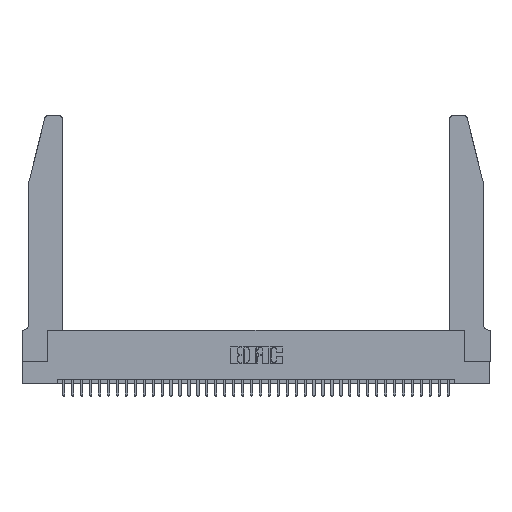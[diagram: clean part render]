
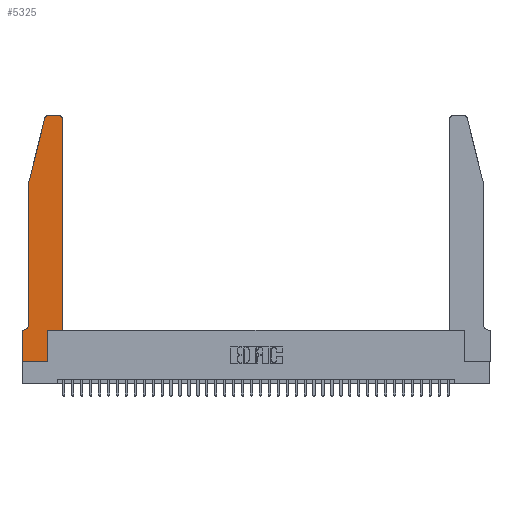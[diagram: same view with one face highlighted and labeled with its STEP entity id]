
A CAD part, top view. The second image highlights one B-rep face of the part: STEP entity #5325.
In plain terms, the highlighted planar face has unit normal (0, 0, 1).
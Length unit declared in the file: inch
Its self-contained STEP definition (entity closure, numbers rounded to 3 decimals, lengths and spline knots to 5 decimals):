
#102 = ORIENTED_EDGE ( 'NONE', *, *, #2865, .T. ) ;
#559 = DIRECTION ( 'NONE',  ( 0., 1., 0. ) ) ;
#920 = CARTESIAN_POINT ( 'NONE',  ( 0.25487, 2.72718, 0.37 ) ) ;
#934 = DIRECTION ( 'NONE',  ( -0.239, -0.971, 0. ) ) ;
#1003 = VECTOR ( 'NONE', #3985, 39.37008 ) ;
#1107 = CARTESIAN_POINT ( 'NONE',  ( 0.2865, 0., 0.37 ) ) ;
#1128 = CARTESIAN_POINT ( 'NONE',  ( 0.2865, 0.35, 0.37 ) ) ;
#1662 = CARTESIAN_POINT ( 'NONE',  ( 0.284, 2.75, 0.37 ) ) ;
#2114 = DIRECTION ( 'NONE',  ( 0., 1., 0. ) ) ;
#2348 = CARTESIAN_POINT ( 'NONE',  ( 0.0755, 2., 0.37 ) ) ;
#2698 = CARTESIAN_POINT ( 'NONE',  ( 0.4505, 2.72, 0.37 ) ) ;
#2772 = CARTESIAN_POINT ( 'NONE',  ( 0.2865, 0.35, 0.37 ) ) ;
#2865 = EDGE_CURVE ( 'NONE', #34028, #33204, #30102, .T. ) ;
#3132 = CARTESIAN_POINT ( 'NONE',  ( 0.0755, 0.42, 0.37 ) ) ;
#3177 = DIRECTION ( 'NONE',  ( -1., 0., 0. ) ) ;
#3985 = DIRECTION ( 'NONE',  ( 1., 0., 0. ) ) ;
#4076 = CARTESIAN_POINT ( 'NONE',  ( 0.284, 2.72, 0.37 ) ) ;
#4104 = DIRECTION ( 'NONE',  ( 1., 0., 0. ) ) ;
#5325 = ADVANCED_FACE ( 'NONE', ( #26105 ), #27949, .T. ) ;
#5665 = EDGE_CURVE ( 'NONE', #29418, #34028, #7273, .T. ) ;
#5741 = DIRECTION ( 'NONE',  ( 0., 0., -1. ) ) ;
#5836 = DIRECTION ( 'NONE',  ( -1., 0., 0. ) ) ;
#6379 = AXIS2_PLACEMENT_3D ( 'NONE', #4076, #25534, #10525 ) ;
#6463 = ORIENTED_EDGE ( 'NONE', *, *, #35112, .T. ) ;
#6534 = LINE ( 'NONE', #32052, #8384 ) ;
#6888 = VERTEX_POINT ( 'NONE', #16538 ) ;
#7093 = LINE ( 'NONE', #21598, #1003 ) ;
#7273 = LINE ( 'NONE', #2772, #18512 ) ;
#7665 = VECTOR ( 'NONE', #18365, 39.37008 ) ;
#8188 = ORIENTED_EDGE ( 'NONE', *, *, #34535, .T. ) ;
#8384 = VECTOR ( 'NONE', #2114, 39.37008 ) ;
#10525 = DIRECTION ( 'NONE',  ( 1., 0., 0. ) ) ;
#11031 = LINE ( 'NONE', #23507, #33711 ) ;
#11554 = ORIENTED_EDGE ( 'NONE', *, *, #23377, .T. ) ;
#12392 = EDGE_CURVE ( 'NONE', #34497, #6888, #34831, .T. ) ;
#12649 = CARTESIAN_POINT ( 'NONE',  ( 0., 0., 0.37 ) ) ;
#12934 = LINE ( 'NONE', #2348, #29475 ) ;
#13133 = EDGE_CURVE ( 'NONE', #25960, #34497, #33866, .T. ) ;
#13815 = CARTESIAN_POINT ( 'NONE',  ( 0.0755, 2., 0.37 ) ) ;
#14030 = AXIS2_PLACEMENT_3D ( 'NONE', #34144, #5741, #27014 ) ;
#14160 = ORIENTED_EDGE ( 'NONE', *, *, #17379, .T. ) ;
#14263 = ORIENTED_EDGE ( 'NONE', *, *, #12392, .T. ) ;
#14401 = CARTESIAN_POINT ( 'NONE',  ( 0.0755, 2., 0.37 ) ) ;
#14428 = EDGE_CURVE ( 'NONE', #38325, #29266, #35371, .T. ) ;
#14585 = ORIENTED_EDGE ( 'NONE', *, *, #14428, .T. ) ;
#14717 = LINE ( 'NONE', #36385, #7665 ) ;
#15028 = CARTESIAN_POINT ( 'NONE',  ( 0.4505, 0.35, 0.37 ) ) ;
#15498 = ORIENTED_EDGE ( 'NONE', *, *, #25316, .T. ) ;
#16071 = DIRECTION ( 'NONE',  ( 0., 0., 1. ) ) ;
#16259 = ORIENTED_EDGE ( 'NONE', *, *, #19610, .T. ) ;
#16538 = CARTESIAN_POINT ( 'NONE',  ( 0.0055, 0.35, 0.37 ) ) ;
#16634 = ORIENTED_EDGE ( 'NONE', *, *, #5665, .T. ) ;
#16711 = EDGE_CURVE ( 'NONE', #36430, #32829, #19089, .T. ) ;
#17379 = EDGE_CURVE ( 'NONE', #32829, #25960, #12934, .T. ) ;
#17958 = LINE ( 'NONE', #33261, #38838 ) ;
#18072 = ORIENTED_EDGE ( 'NONE', *, *, #13133, .T. ) ;
#18365 = DIRECTION ( 'NONE',  ( 0., -1., 0. ) ) ;
#18512 = VECTOR ( 'NONE', #559, 39.37008 ) ;
#18659 = CARTESIAN_POINT ( 'NONE',  ( 0., 0.35, 0.37 ) ) ;
#19089 = CIRCLE ( 'NONE', #6379, 0.03 ) ;
#19610 = EDGE_CURVE ( 'NONE', #33850, #29418, #7093, .T. ) ;
#19843 = EDGE_LOOP ( 'NONE', ( #6463, #31378, #14160, #18072, #14263, #15498, #8188, #16259, #16634, #102, #11554, #14585 ) ) ;
#21170 = CARTESIAN_POINT ( 'NONE',  ( 0.4205, 2.75, 0.37 ) ) ;
#21199 = DIRECTION ( 'NONE',  ( 1., 0., 0. ) ) ;
#21598 = CARTESIAN_POINT ( 'NONE',  ( 0., 0., 0.37 ) ) ;
#23377 = EDGE_CURVE ( 'NONE', #33204, #38325, #6534, .T. ) ;
#23507 = CARTESIAN_POINT ( 'NONE',  ( 0.0755, 0.35, 0.37 ) ) ;
#24475 = AXIS2_PLACEMENT_3D ( 'NONE', #18659, #24754, #30709 ) ;
#24754 = DIRECTION ( 'NONE',  ( 0., 0., 1. ) ) ;
#25316 = EDGE_CURVE ( 'NONE', #6888, #27451, #11031, .T. ) ;
#25534 = DIRECTION ( 'NONE',  ( 0., 0., 1. ) ) ;
#25960 = VERTEX_POINT ( 'NONE', #14401 ) ;
#26105 = FACE_OUTER_BOUND ( 'NONE', #19843, .T. ) ;
#26129 = CARTESIAN_POINT ( 'NONE',  ( 0.4505, 0.35, 0.37 ) ) ;
#26995 = AXIS2_PLACEMENT_3D ( 'NONE', #34210, #16071, #4104 ) ;
#27014 = DIRECTION ( 'NONE',  ( -1., 0., 0. ) ) ;
#27451 = VERTEX_POINT ( 'NONE', #28506 ) ;
#27949 = PLANE ( 'NONE',  #24475 ) ;
#28196 = VECTOR ( 'NONE', #29269, 39.37008 ) ;
#28506 = CARTESIAN_POINT ( 'NONE',  ( 0., 0.35, 0.37 ) ) ;
#29266 = VERTEX_POINT ( 'NONE', #21170 ) ;
#29269 = DIRECTION ( 'NONE',  ( 0., -1., 0. ) ) ;
#29418 = VERTEX_POINT ( 'NONE', #1107 ) ;
#29475 = VECTOR ( 'NONE', #934, 39.37008 ) ;
#30102 = LINE ( 'NONE', #15028, #34863 ) ;
#30709 = DIRECTION ( 'NONE',  ( 1., 0., 0. ) ) ;
#31378 = ORIENTED_EDGE ( 'NONE', *, *, #16711, .T. ) ;
#32052 = CARTESIAN_POINT ( 'NONE',  ( 0.4505, 0.35, 0.37 ) ) ;
#32829 = VERTEX_POINT ( 'NONE', #920 ) ;
#33204 = VERTEX_POINT ( 'NONE', #26129 ) ;
#33261 = CARTESIAN_POINT ( 'NONE',  ( 0.2605, 2.75, 0.37 ) ) ;
#33711 = VECTOR ( 'NONE', #5836, 39.37008 ) ;
#33850 = VERTEX_POINT ( 'NONE', #12649 ) ;
#33866 = LINE ( 'NONE', #13815, #28196 ) ;
#34028 = VERTEX_POINT ( 'NONE', #1128 ) ;
#34144 = CARTESIAN_POINT ( 'NONE',  ( 0.0055, 0.42, 0.37 ) ) ;
#34210 = CARTESIAN_POINT ( 'NONE',  ( 0.4205, 2.72, 0.37 ) ) ;
#34497 = VERTEX_POINT ( 'NONE', #3132 ) ;
#34535 = EDGE_CURVE ( 'NONE', #27451, #33850, #14717, .T. ) ;
#34831 = CIRCLE ( 'NONE', #14030, 0.07 ) ;
#34863 = VECTOR ( 'NONE', #21199, 39.37008 ) ;
#35112 = EDGE_CURVE ( 'NONE', #29266, #36430, #17958, .T. ) ;
#35371 = CIRCLE ( 'NONE', #26995, 0.03 ) ;
#36385 = CARTESIAN_POINT ( 'NONE',  ( 0., 0., 0.37 ) ) ;
#36430 = VERTEX_POINT ( 'NONE', #1662 ) ;
#38325 = VERTEX_POINT ( 'NONE', #2698 ) ;
#38838 = VECTOR ( 'NONE', #3177, 39.37008 ) ;
